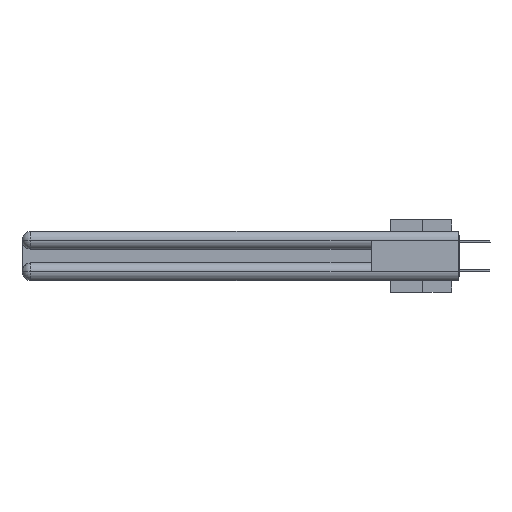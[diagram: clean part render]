
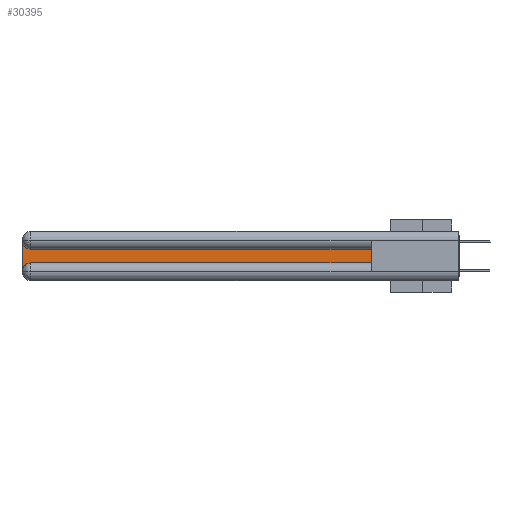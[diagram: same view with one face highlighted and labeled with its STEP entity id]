
A CAD part, left-side view. The second image highlights one B-rep face of the part: STEP entity #30395.
In plain terms, the highlighted planar face has unit normal (-1, 0, 0).
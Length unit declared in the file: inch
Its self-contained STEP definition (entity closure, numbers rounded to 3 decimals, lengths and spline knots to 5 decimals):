
#576 = VECTOR ( 'NONE', #14836, 39.37008 ) ;
#746 = FACE_OUTER_BOUND ( 'NONE', #26933, .T. ) ;
#2124 = DIRECTION ( 'NONE',  ( 0., 0., -1. ) ) ;
#2331 = VERTEX_POINT ( 'NONE', #11203 ) ;
#2889 = CARTESIAN_POINT ( 'NONE',  ( 0.075, 3., -0.1225 ) ) ;
#3956 = CARTESIAN_POINT ( 'NONE',  ( 0.075, 0.6, -0.2175 ) ) ;
#5519 = AXIS2_PLACEMENT_3D ( 'NONE', #6565, #17473, #28441 ) ;
#5544 = CARTESIAN_POINT ( 'NONE',  ( 0.075, 3., -0.2775 ) ) ;
#5767 = CARTESIAN_POINT ( 'NONE',  ( 0.075, 2.94, -0.1225 ) ) ;
#6203 = VERTEX_POINT ( 'NONE', #5544 ) ;
#6565 = CARTESIAN_POINT ( 'NONE',  ( 0.075, 2.94, -0.2775 ) ) ;
#6930 = VECTOR ( 'NONE', #8587, 39.37008 ) ;
#7030 = CARTESIAN_POINT ( 'NONE',  ( 0.075, 2.94, -0.2175 ) ) ;
#7810 = EDGE_CURVE ( 'NONE', #31146, #26075, #29858, .T. ) ;
#8187 = ORIENTED_EDGE ( 'NONE', *, *, #9321, .T. ) ;
#8364 = CIRCLE ( 'NONE', #5519, 0.06 ) ;
#8495 = CARTESIAN_POINT ( 'NONE',  ( 0.075, 0.6, -0.2175 ) ) ;
#8587 = DIRECTION ( 'NONE',  ( 0., 0., -1. ) ) ;
#9321 = EDGE_CURVE ( 'NONE', #6203, #24522, #8364, .T. ) ;
#9679 = CARTESIAN_POINT ( 'NONE',  ( 0.075, 0.6, -0.2175 ) ) ;
#11203 = CARTESIAN_POINT ( 'NONE',  ( 0.075, 3., -0.0625 ) ) ;
#11565 = ORIENTED_EDGE ( 'NONE', *, *, #20076, .T. ) ;
#12494 = AXIS2_PLACEMENT_3D ( 'NONE', #17861, #15694, #2124 ) ;
#13772 = PLANE ( 'NONE',  #35008 ) ;
#13893 = DIRECTION ( 'NONE',  ( 0., 1., 0. ) ) ;
#14836 = DIRECTION ( 'NONE',  ( 0., 0., 1. ) ) ;
#15694 = DIRECTION ( 'NONE',  ( 1., 0., 0. ) ) ;
#17129 = EDGE_CURVE ( 'NONE', #26075, #2331, #33761, .T. ) ;
#17473 = DIRECTION ( 'NONE',  ( 1., 0., 0. ) ) ;
#17861 = CARTESIAN_POINT ( 'NONE',  ( 0.075, 2.94, -0.0625 ) ) ;
#18325 = EDGE_CURVE ( 'NONE', #24979, #31146, #20235, .T. ) ;
#18475 = ORIENTED_EDGE ( 'NONE', *, *, #22214, .T. ) ;
#18725 = CARTESIAN_POINT ( 'NONE',  ( 0.075, 0.6, -0.1225 ) ) ;
#18890 = LINE ( 'NONE', #8495, #28810 ) ;
#19885 = DIRECTION ( 'NONE',  ( 0., 0., -1. ) ) ;
#20000 = ORIENTED_EDGE ( 'NONE', *, *, #18325, .T. ) ;
#20076 = EDGE_CURVE ( 'NONE', #2331, #6203, #24723, .T. ) ;
#20235 = LINE ( 'NONE', #3956, #576 ) ;
#22214 = EDGE_CURVE ( 'NONE', #24522, #24979, #18890, .T. ) ;
#22400 = CARTESIAN_POINT ( 'NONE',  ( 0.075, 3., -0.2175 ) ) ;
#24522 = VERTEX_POINT ( 'NONE', #7030 ) ;
#24723 = LINE ( 'NONE', #22400, #6930 ) ;
#24979 = VERTEX_POINT ( 'NONE', #9679 ) ;
#25473 = VECTOR ( 'NONE', #13893, 39.37008 ) ;
#26075 = VERTEX_POINT ( 'NONE', #5767 ) ;
#26933 = EDGE_LOOP ( 'NONE', ( #31150, #28578, #11565, #8187, #18475, #20000 ) ) ;
#28441 = DIRECTION ( 'NONE',  ( 0., 0., -1. ) ) ;
#28578 = ORIENTED_EDGE ( 'NONE', *, *, #17129, .T. ) ;
#28810 = VECTOR ( 'NONE', #32869, 39.37008 ) ;
#29858 = LINE ( 'NONE', #35062, #25473 ) ;
#30395 = ADVANCED_FACE ( 'NONE', ( #746 ), #13772, .F. ) ;
#31146 = VERTEX_POINT ( 'NONE', #18725 ) ;
#31150 = ORIENTED_EDGE ( 'NONE', *, *, #7810, .T. ) ;
#32869 = DIRECTION ( 'NONE',  ( 0., -1., 0. ) ) ;
#33324 = DIRECTION ( 'NONE',  ( 1., 0., 0. ) ) ;
#33761 = CIRCLE ( 'NONE', #12494, 0.06 ) ;
#35008 = AXIS2_PLACEMENT_3D ( 'NONE', #2889, #33324, #19885 ) ;
#35062 = CARTESIAN_POINT ( 'NONE',  ( 0.075, 0.6, -0.1225 ) ) ;
